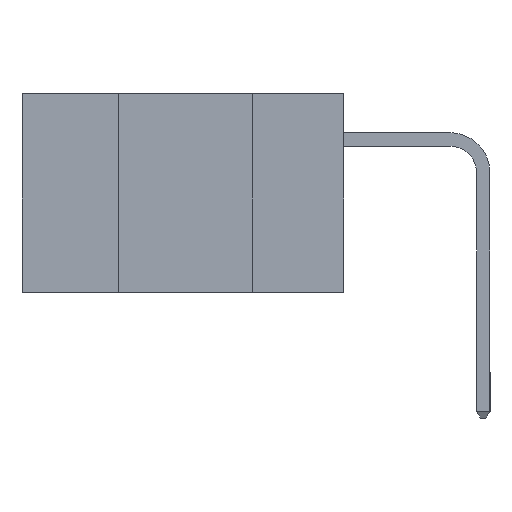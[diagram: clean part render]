
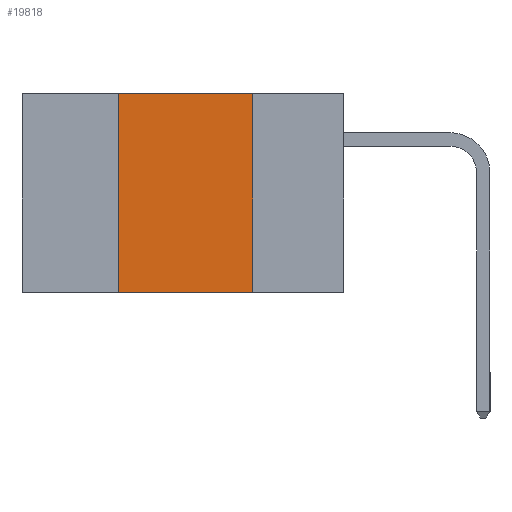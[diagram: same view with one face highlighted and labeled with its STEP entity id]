
A CAD part, left-side view. The second image highlights one B-rep face of the part: STEP entity #19818.
In plain terms, the highlighted planar face has unit normal (-1, 0, 0).
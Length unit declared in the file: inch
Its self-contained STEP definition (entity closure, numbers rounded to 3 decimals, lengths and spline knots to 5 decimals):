
#269 = AXIS2_PLACEMENT_3D ( 'NONE', #9141, #7568, #6713 ) ;
#756 = VECTOR ( 'NONE', #16580, 39.37008 ) ;
#1140 = LINE ( 'NONE', #12518, #2956 ) ;
#1926 = VERTEX_POINT ( 'NONE', #20645 ) ;
#1978 = VERTEX_POINT ( 'NONE', #9550 ) ;
#2896 = DIRECTION ( 'NONE',  ( 0., 0., 1. ) ) ;
#2956 = VECTOR ( 'NONE', #20322, 39.37008 ) ;
#3822 = LINE ( 'NONE', #9950, #756 ) ;
#6614 = VECTOR ( 'NONE', #2896, 39.37008 ) ;
#6713 = DIRECTION ( 'NONE',  ( 0., 0., -1. ) ) ;
#7168 = ORIENTED_EDGE ( 'NONE', *, *, #7665, .T. ) ;
#7568 = DIRECTION ( 'NONE',  ( 1., 0., 0. ) ) ;
#7665 = EDGE_CURVE ( 'NONE', #1978, #1926, #3822, .T. ) ;
#7931 = CARTESIAN_POINT ( 'NONE',  ( 0., 0.42, 0. ) ) ;
#8236 = VERTEX_POINT ( 'NONE', #17650 ) ;
#9044 = FACE_OUTER_BOUND ( 'NONE', #9482, .T. ) ;
#9141 = CARTESIAN_POINT ( 'NONE',  ( 0., 0.6, 0. ) ) ;
#9415 = EDGE_CURVE ( 'NONE', #8236, #1926, #13057, .T. ) ;
#9482 = EDGE_LOOP ( 'NONE', ( #14350, #12326, #11622, #7168 ) ) ;
#9550 = CARTESIAN_POINT ( 'NONE',  ( 0., 0.42, -0.37 ) ) ;
#9950 = CARTESIAN_POINT ( 'NONE',  ( 0., 0.6, -0.37 ) ) ;
#10026 = VERTEX_POINT ( 'NONE', #7931 ) ;
#11116 = CARTESIAN_POINT ( 'NONE',  ( 0., 0.42, -0.37 ) ) ;
#11622 = ORIENTED_EDGE ( 'NONE', *, *, #18506, .F. ) ;
#12326 = ORIENTED_EDGE ( 'NONE', *, *, #19707, .F. ) ;
#12518 = CARTESIAN_POINT ( 'NONE',  ( 0., 0.6, 0. ) ) ;
#12596 = LINE ( 'NONE', #11116, #6614 ) ;
#13057 = LINE ( 'NONE', #17904, #15262 ) ;
#14350 = ORIENTED_EDGE ( 'NONE', *, *, #9415, .F. ) ;
#15262 = VECTOR ( 'NONE', #16315, 39.37008 ) ;
#16315 = DIRECTION ( 'NONE',  ( 0., 0., -1. ) ) ;
#16580 = DIRECTION ( 'NONE',  ( 0., -1., 0. ) ) ;
#17176 = PLANE ( 'NONE',  #269 ) ;
#17650 = CARTESIAN_POINT ( 'NONE',  ( 0., 0.17, 0. ) ) ;
#17904 = CARTESIAN_POINT ( 'NONE',  ( 0., 0.17, -0.37 ) ) ;
#18506 = EDGE_CURVE ( 'NONE', #1978, #10026, #12596, .T. ) ;
#19707 = EDGE_CURVE ( 'NONE', #10026, #8236, #1140, .T. ) ;
#19818 = ADVANCED_FACE ( 'NONE', ( #9044 ), #17176, .F. ) ;
#20322 = DIRECTION ( 'NONE',  ( 0., -1., 0. ) ) ;
#20645 = CARTESIAN_POINT ( 'NONE',  ( 0., 0.17, -0.37 ) ) ;
